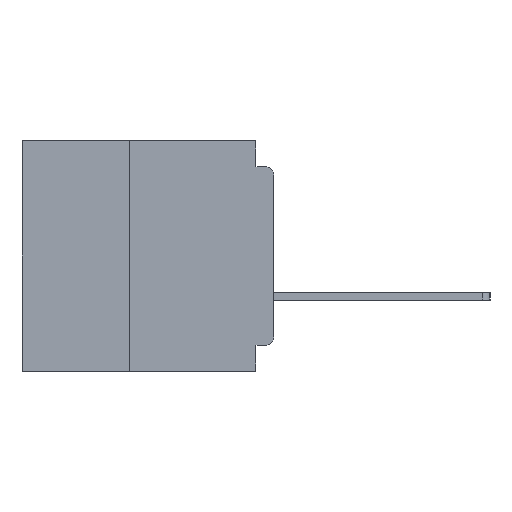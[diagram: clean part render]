
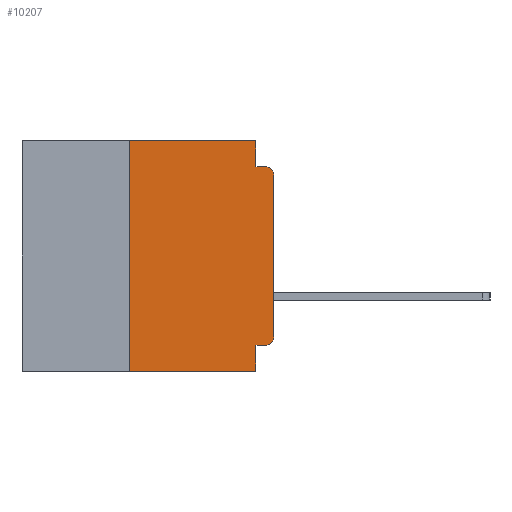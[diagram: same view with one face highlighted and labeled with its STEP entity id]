
A CAD part, left-side view. The second image highlights one B-rep face of the part: STEP entity #10207.
In plain terms, the highlighted planar face has unit normal (-1, 0, 0).
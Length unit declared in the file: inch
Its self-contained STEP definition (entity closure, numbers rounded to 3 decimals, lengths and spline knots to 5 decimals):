
#107 = CARTESIAN_POINT ( 'NONE',  ( 0., 0.25, -0.4 ) ) ;
#917 = VERTEX_POINT ( 'NONE', #107 ) ;
#1102 = DIRECTION ( 'NONE',  ( 0., 0., -1. ) ) ;
#1286 = CARTESIAN_POINT ( 'NONE',  ( 0., 0.031, 0. ) ) ;
#1767 = VERTEX_POINT ( 'NONE', #25383 ) ;
#1797 = VECTOR ( 'NONE', #19672, 39.37008 ) ;
#2074 = ORIENTED_EDGE ( 'NONE', *, *, #3626, .T. ) ;
#2126 = ORIENTED_EDGE ( 'NONE', *, *, #6734, .T. ) ;
#2329 = CARTESIAN_POINT ( 'NONE',  ( 0., 0.437, 0. ) ) ;
#2499 = DIRECTION ( 'NONE',  ( 0., 0., -1. ) ) ;
#2969 = VECTOR ( 'NONE', #10355, 39.37008 ) ;
#3626 = EDGE_CURVE ( 'NONE', #917, #15306, #23055, .T. ) ;
#3674 = VERTEX_POINT ( 'NONE', #26696 ) ;
#4499 = DIRECTION ( 'NONE',  ( 0., 0., 1. ) ) ;
#4777 = VERTEX_POINT ( 'NONE', #27500 ) ;
#4946 = CARTESIAN_POINT ( 'NONE',  ( 0., 0.031, 0. ) ) ;
#5355 = VECTOR ( 'NONE', #8393, 39.37008 ) ;
#5688 = CARTESIAN_POINT ( 'NONE',  ( 0., 0.25, -0.4 ) ) ;
#6336 = CARTESIAN_POINT ( 'NONE',  ( 0., 0.015, -0.355 ) ) ;
#6734 = EDGE_CURVE ( 'NONE', #13013, #1767, #39477, .T. ) ;
#7373 = CIRCLE ( 'NONE', #20255, 0.015 ) ;
#7441 = ORIENTED_EDGE ( 'NONE', *, *, #10762, .F. ) ;
#8021 = DIRECTION ( 'NONE',  ( 1., 0., 0. ) ) ;
#8393 = DIRECTION ( 'NONE',  ( 0., 0., -1. ) ) ;
#8713 = VERTEX_POINT ( 'NONE', #6336 ) ;
#8795 = VECTOR ( 'NONE', #12633, 39.37008 ) ;
#10207 = ADVANCED_FACE ( 'NONE', ( #22816 ), #28340, .F. ) ;
#10355 = DIRECTION ( 'NONE',  ( 0., 0., -1. ) ) ;
#10608 = VECTOR ( 'NONE', #37684, 39.37008 ) ;
#10762 = EDGE_CURVE ( 'NONE', #8713, #23129, #28582, .T. ) ;
#10975 = VERTEX_POINT ( 'NONE', #35497 ) ;
#11174 = AXIS2_PLACEMENT_3D ( 'NONE', #42797, #22853, #2499 ) ;
#12633 = DIRECTION ( 'NONE',  ( 0., -1., 0. ) ) ;
#13013 = VERTEX_POINT ( 'NONE', #20048 ) ;
#15306 = VERTEX_POINT ( 'NONE', #19565 ) ;
#15959 = DIRECTION ( 'NONE',  ( 0., 0., 1. ) ) ;
#17144 = CARTESIAN_POINT ( 'NONE',  ( 0., 0.031, -0.355 ) ) ;
#17541 = CARTESIAN_POINT ( 'NONE',  ( 0., 0., -0.355 ) ) ;
#17799 = LINE ( 'NONE', #2329, #8795 ) ;
#18121 = CARTESIAN_POINT ( 'NONE',  ( 0., 0.437, 0. ) ) ;
#19565 = CARTESIAN_POINT ( 'NONE',  ( 0., 0.031, -0.4 ) ) ;
#19672 = DIRECTION ( 'NONE',  ( 0., -1., 0. ) ) ;
#20048 = CARTESIAN_POINT ( 'NONE',  ( 0., 0., -0.34 ) ) ;
#20255 = AXIS2_PLACEMENT_3D ( 'NONE', #41455, #21475, #1102 ) ;
#21065 = LINE ( 'NONE', #37269, #2969 ) ;
#21442 = CARTESIAN_POINT ( 'NONE',  ( 0., 0., 0. ) ) ;
#21475 = DIRECTION ( 'NONE',  ( -1., 0., 0. ) ) ;
#21700 = VECTOR ( 'NONE', #4499, 39.37008 ) ;
#22816 = FACE_OUTER_BOUND ( 'NONE', #40083, .T. ) ;
#22853 = DIRECTION ( 'NONE',  ( -1., 0., 0. ) ) ;
#23055 = LINE ( 'NONE', #28658, #38733 ) ;
#23129 = VERTEX_POINT ( 'NONE', #17144 ) ;
#24171 = EDGE_CURVE ( 'NONE', #10975, #27829, #17799, .T. ) ;
#24425 = ORIENTED_EDGE ( 'NONE', *, *, #36196, .F. ) ;
#25383 = CARTESIAN_POINT ( 'NONE',  ( 0., 0., -0.06 ) ) ;
#26696 = CARTESIAN_POINT ( 'NONE',  ( 0., 0.031, -0.045 ) ) ;
#27273 = LINE ( 'NONE', #5688, #35130 ) ;
#27500 = CARTESIAN_POINT ( 'NONE',  ( 0., 0.015, -0.045 ) ) ;
#27829 = VERTEX_POINT ( 'NONE', #1286 ) ;
#28108 = ORIENTED_EDGE ( 'NONE', *, *, #28651, .F. ) ;
#28340 = PLANE ( 'NONE',  #35285 ) ;
#28582 = LINE ( 'NONE', #17541, #10608 ) ;
#28651 = EDGE_CURVE ( 'NONE', #917, #10975, #27273, .T. ) ;
#28658 = CARTESIAN_POINT ( 'NONE',  ( 0., 0.437, -0.4 ) ) ;
#30372 = DIRECTION ( 'NONE',  ( 0., -1., 0. ) ) ;
#30879 = EDGE_CURVE ( 'NONE', #27829, #3674, #32355, .T. ) ;
#31692 = DIRECTION ( 'NONE',  ( 0., 0., -1. ) ) ;
#32355 = LINE ( 'NONE', #4946, #5355 ) ;
#33841 = ORIENTED_EDGE ( 'NONE', *, *, #24171, .F. ) ;
#34202 = EDGE_CURVE ( 'NONE', #1767, #4777, #7373, .T. ) ;
#35130 = VECTOR ( 'NONE', #15959, 39.37008 ) ;
#35285 = AXIS2_PLACEMENT_3D ( 'NONE', #18121, #8021, #31692 ) ;
#35497 = CARTESIAN_POINT ( 'NONE',  ( 0., 0.25, 0. ) ) ;
#36196 = EDGE_CURVE ( 'NONE', #23129, #15306, #21065, .T. ) ;
#36459 = CIRCLE ( 'NONE', #11174, 0.015 ) ;
#36482 = ORIENTED_EDGE ( 'NONE', *, *, #40979, .T. ) ;
#36704 = LINE ( 'NONE', #39724, #1797 ) ;
#37269 = CARTESIAN_POINT ( 'NONE',  ( 0., 0.031, -0.4 ) ) ;
#37684 = DIRECTION ( 'NONE',  ( 0., 1., 0. ) ) ;
#37827 = EDGE_CURVE ( 'NONE', #3674, #4777, #36704, .T. ) ;
#38057 = ORIENTED_EDGE ( 'NONE', *, *, #34202, .T. ) ;
#38733 = VECTOR ( 'NONE', #30372, 39.37008 ) ;
#39477 = LINE ( 'NONE', #21442, #21700 ) ;
#39724 = CARTESIAN_POINT ( 'NONE',  ( 0., 0., -0.045 ) ) ;
#40083 = EDGE_LOOP ( 'NONE', ( #2126, #38057, #40113, #41144, #33841, #28108, #2074, #24425, #7441, #36482 ) ) ;
#40113 = ORIENTED_EDGE ( 'NONE', *, *, #37827, .F. ) ;
#40979 = EDGE_CURVE ( 'NONE', #8713, #13013, #36459, .T. ) ;
#41144 = ORIENTED_EDGE ( 'NONE', *, *, #30879, .F. ) ;
#41455 = CARTESIAN_POINT ( 'NONE',  ( 0., 0.015, -0.06 ) ) ;
#42797 = CARTESIAN_POINT ( 'NONE',  ( 0., 0.015, -0.34 ) ) ;
